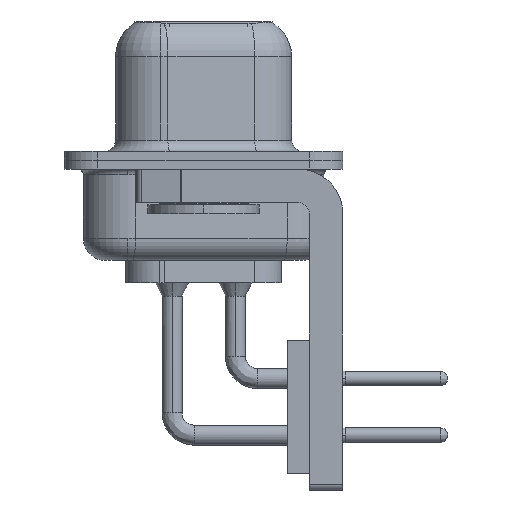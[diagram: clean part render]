
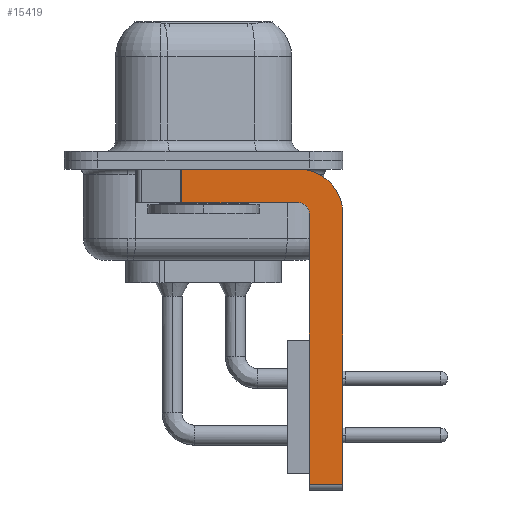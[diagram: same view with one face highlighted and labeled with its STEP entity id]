
A CAD part, left-side view. The second image highlights one B-rep face of the part: STEP entity #15419.
In plain terms, the highlighted planar face has unit normal (-1, 0, 0).
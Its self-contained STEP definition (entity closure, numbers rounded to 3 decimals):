
#94 = DIRECTION ( 'NONE',  ( 0., -1., 0. ) ) ;
#245 = ORIENTED_EDGE ( 'NONE', *, *, #10101, .F. ) ;
#413 = ORIENTED_EDGE ( 'NONE', *, *, #13311, .F. ) ;
#421 = ORIENTED_EDGE ( 'NONE', *, *, #14931, .F. ) ;
#1013 = CIRCLE ( 'NONE', #13235, 2. ) ;
#1172 = CIRCLE ( 'NONE', #11053, 0.5 ) ;
#1516 = AXIS2_PLACEMENT_3D ( 'NONE', #3254, #3334, #16871 ) ;
#1589 = CARTESIAN_POINT ( 'NONE',  ( -2.9, 0.978, -1.9 ) ) ;
#1715 = EDGE_CURVE ( 'NONE', #3976, #23365, #1013, .T. ) ;
#2403 = EDGE_CURVE ( 'NONE', #14491, #3805, #17834, .T. ) ;
#2518 = DIRECTION ( 'NONE',  ( 0., 0., 1. ) ) ;
#2675 = VERTEX_POINT ( 'NONE', #3813 ) ;
#3002 = CARTESIAN_POINT ( 'NONE',  ( -2.9, -4.75, -2.4 ) ) ;
#3254 = CARTESIAN_POINT ( 'NONE',  ( -2.9, -4.25, -2.4 ) ) ;
#3334 = DIRECTION ( 'NONE',  ( 1., 0., 0. ) ) ;
#3805 = VERTEX_POINT ( 'NONE', #1589 ) ;
#3813 = CARTESIAN_POINT ( 'NONE',  ( -2.9, -6.25, -14.55 ) ) ;
#3864 = CARTESIAN_POINT ( 'NONE',  ( -2.9, 3., -0.4 ) ) ;
#3976 = VERTEX_POINT ( 'NONE', #14412 ) ;
#4161 = LINE ( 'NONE', #13876, #8132 ) ;
#5308 = ORIENTED_EDGE ( 'NONE', *, *, #7271, .F. ) ;
#5354 = DIRECTION ( 'NONE',  ( -1., 0., 0. ) ) ;
#5579 = EDGE_CURVE ( 'NONE', #17106, #2675, #9913, .T. ) ;
#6770 = DIRECTION ( 'NONE',  ( 0., -1., 0. ) ) ;
#7013 = CARTESIAN_POINT ( 'NONE',  ( -2.9, -4.25, -1.9 ) ) ;
#7191 = PLANE ( 'NONE',  #1516 ) ;
#7271 = EDGE_CURVE ( 'NONE', #17106, #14297, #24645, .T. ) ;
#7839 = FACE_OUTER_BOUND ( 'NONE', #9280, .T. ) ;
#8099 = CARTESIAN_POINT ( 'NONE',  ( -2.9, -4.75, -14.8 ) ) ;
#8132 = VECTOR ( 'NONE', #17607, 1000. ) ;
#9105 = DIRECTION ( 'NONE',  ( 0., 0., -1. ) ) ;
#9280 = EDGE_LOOP ( 'NONE', ( #421, #18619, #24827, #413, #5308, #9537, #245, #14974 ) ) ;
#9537 = ORIENTED_EDGE ( 'NONE', *, *, #5579, .T. ) ;
#9913 = LINE ( 'NONE', #10867, #24719 ) ;
#10101 = EDGE_CURVE ( 'NONE', #23365, #2675, #19859, .T. ) ;
#10301 = CARTESIAN_POINT ( 'NONE',  ( -2.9, 0.978, -1.9 ) ) ;
#10867 = CARTESIAN_POINT ( 'NONE',  ( -2.9, -4.25, -14.55 ) ) ;
#11053 = AXIS2_PLACEMENT_3D ( 'NONE', #16953, #5354, #18819 ) ;
#11239 = VECTOR ( 'NONE', #94, 1000. ) ;
#11880 = LINE ( 'NONE', #3864, #11239 ) ;
#13235 = AXIS2_PLACEMENT_3D ( 'NONE', #21017, #21013, #17043 ) ;
#13311 = EDGE_CURVE ( 'NONE', #14297, #14305, #1172, .T. ) ;
#13876 = CARTESIAN_POINT ( 'NONE',  ( -2.9, -4.25, -1.9 ) ) ;
#14297 = VERTEX_POINT ( 'NONE', #3002 ) ;
#14305 = VERTEX_POINT ( 'NONE', #7013 ) ;
#14412 = CARTESIAN_POINT ( 'NONE',  ( -2.9, -4.25, -0.4 ) ) ;
#14491 = VERTEX_POINT ( 'NONE', #20885 ) ;
#14917 = VECTOR ( 'NONE', #15057, 1000. ) ;
#14931 = EDGE_CURVE ( 'NONE', #14491, #3976, #11880, .T. ) ;
#14974 = ORIENTED_EDGE ( 'NONE', *, *, #1715, .F. ) ;
#15057 = DIRECTION ( 'NONE',  ( 0., 0., -1. ) ) ;
#15419 = ADVANCED_FACE ( 'NONE', ( #7839 ), #7191, .F. ) ;
#15688 = EDGE_CURVE ( 'NONE', #14305, #3805, #4161, .T. ) ;
#16871 = DIRECTION ( 'NONE',  ( 0., 0., -1. ) ) ;
#16953 = CARTESIAN_POINT ( 'NONE',  ( -2.9, -4.25, -2.4 ) ) ;
#17043 = DIRECTION ( 'NONE',  ( 0., 0., -1. ) ) ;
#17106 = VERTEX_POINT ( 'NONE', #22652 ) ;
#17607 = DIRECTION ( 'NONE',  ( 0., 1., 0. ) ) ;
#17834 = LINE ( 'NONE', #10301, #18400 ) ;
#18400 = VECTOR ( 'NONE', #9105, 1000. ) ;
#18619 = ORIENTED_EDGE ( 'NONE', *, *, #2403, .T. ) ;
#18819 = DIRECTION ( 'NONE',  ( 0., 0., 1. ) ) ;
#19374 = VECTOR ( 'NONE', #2518, 1000. ) ;
#19859 = LINE ( 'NONE', #22571, #14917 ) ;
#20885 = CARTESIAN_POINT ( 'NONE',  ( -2.9, 0.978, -0.4 ) ) ;
#21013 = DIRECTION ( 'NONE',  ( 1., 0., 0. ) ) ;
#21017 = CARTESIAN_POINT ( 'NONE',  ( -2.9, -4.25, -2.4 ) ) ;
#21291 = CARTESIAN_POINT ( 'NONE',  ( -2.9, -6.25, -2.4 ) ) ;
#22571 = CARTESIAN_POINT ( 'NONE',  ( -2.9, -6.25, -2.4 ) ) ;
#22652 = CARTESIAN_POINT ( 'NONE',  ( -2.9, -4.75, -14.55 ) ) ;
#23365 = VERTEX_POINT ( 'NONE', #21291 ) ;
#24645 = LINE ( 'NONE', #8099, #19374 ) ;
#24719 = VECTOR ( 'NONE', #6770, 1000. ) ;
#24827 = ORIENTED_EDGE ( 'NONE', *, *, #15688, .F. ) ;
